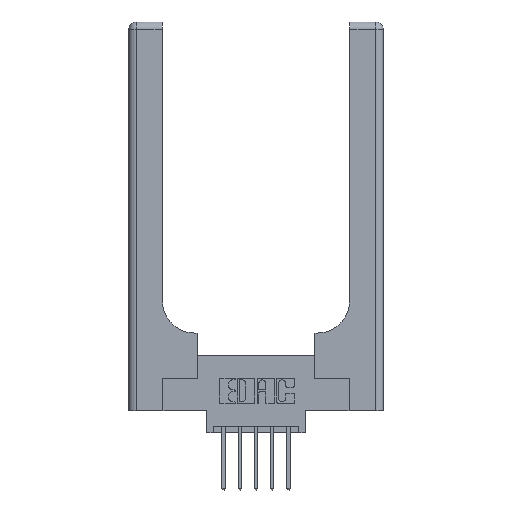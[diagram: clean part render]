
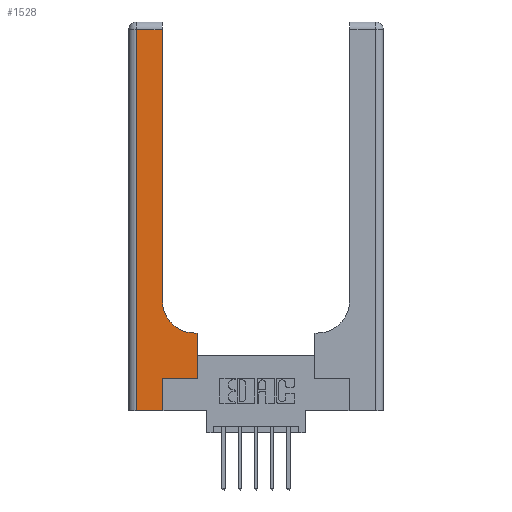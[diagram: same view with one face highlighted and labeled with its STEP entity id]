
A CAD part, top view. The second image highlights one B-rep face of the part: STEP entity #1528.
In plain terms, the highlighted planar face has unit normal (0, 0, 1).
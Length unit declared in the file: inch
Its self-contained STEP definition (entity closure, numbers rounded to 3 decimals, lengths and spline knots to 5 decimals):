
#241 = VERTEX_POINT ( 'NONE', #13091 ) ;
#368 = CARTESIAN_POINT ( 'NONE',  ( 0.26, 0.6, 0.37 ) ) ;
#558 = AXIS2_PLACEMENT_3D ( 'NONE', #2887, #4079, #7356 ) ;
#729 = EDGE_CURVE ( 'NONE', #6492, #241, #1515, .T. ) ;
#746 = EDGE_CURVE ( 'NONE', #5342, #8816, #9026, .T. ) ;
#931 = VECTOR ( 'NONE', #11128, 39.37008 ) ;
#939 = VERTEX_POINT ( 'NONE', #9441 ) ;
#1125 = CARTESIAN_POINT ( 'NONE',  ( 0., 2.94, 0.37 ) ) ;
#1515 = LINE ( 'NONE', #6970, #931 ) ;
#1528 = ADVANCED_FACE ( 'NONE', ( #13864 ), #2510, .F. ) ;
#1964 = LINE ( 'NONE', #7212, #5113 ) ;
#2036 = DIRECTION ( 'NONE',  ( 0., 0., -1. ) ) ;
#2058 = CARTESIAN_POINT ( 'NONE',  ( 0.06, 3., 0.37 ) ) ;
#2380 = CARTESIAN_POINT ( 'NONE',  ( 0.26, 3., 0.37 ) ) ;
#2453 = EDGE_CURVE ( 'NONE', #11182, #13626, #10834, .T. ) ;
#2510 = PLANE ( 'NONE',  #11345 ) ;
#2789 = EDGE_LOOP ( 'NONE', ( #8010, #5596, #9227, #6378, #9759, #4719, #12224, #5224, #10819 ) ) ;
#2887 = CARTESIAN_POINT ( 'NONE',  ( 0.51, 0.85, 0.37 ) ) ;
#4079 = DIRECTION ( 'NONE',  ( 0., 0., -1. ) ) ;
#4421 = EDGE_CURVE ( 'NONE', #13109, #10190, #1964, .T. ) ;
#4426 = CARTESIAN_POINT ( 'NONE',  ( 0.265, 0., 0.37 ) ) ;
#4457 = CARTESIAN_POINT ( 'NONE',  ( 0.51, 0.6, 0.37 ) ) ;
#4687 = EDGE_CURVE ( 'NONE', #939, #11182, #5651, .T. ) ;
#4712 = DIRECTION ( 'NONE',  ( 0., 1., 0. ) ) ;
#4719 = ORIENTED_EDGE ( 'NONE', *, *, #729, .T. ) ;
#4799 = VECTOR ( 'NONE', #5470, 39.37008 ) ;
#5113 = VECTOR ( 'NONE', #13652, 39.37008 ) ;
#5189 = CARTESIAN_POINT ( 'NONE',  ( 0.06, 0., 0.37 ) ) ;
#5224 = ORIENTED_EDGE ( 'NONE', *, *, #746, .T. ) ;
#5342 = VERTEX_POINT ( 'NONE', #6274 ) ;
#5470 = DIRECTION ( 'NONE',  ( 0., -1., 0. ) ) ;
#5596 = ORIENTED_EDGE ( 'NONE', *, *, #2453, .T. ) ;
#5651 = LINE ( 'NONE', #2380, #13481 ) ;
#5826 = DIRECTION ( 'NONE',  ( -1., 0., 0. ) ) ;
#6274 = CARTESIAN_POINT ( 'NONE',  ( 0.528, 0.6, 0.37 ) ) ;
#6378 = ORIENTED_EDGE ( 'NONE', *, *, #4421, .T. ) ;
#6492 = VERTEX_POINT ( 'NONE', #9311 ) ;
#6605 = LINE ( 'NONE', #12118, #6764 ) ;
#6692 = CIRCLE ( 'NONE', #558, 0.25 ) ;
#6764 = VECTOR ( 'NONE', #10903, 39.37008 ) ;
#6970 = CARTESIAN_POINT ( 'NONE',  ( 0.265, 0.25, 0.37 ) ) ;
#7134 = EDGE_CURVE ( 'NONE', #10190, #6492, #11827, .T. ) ;
#7212 = CARTESIAN_POINT ( 'NONE',  ( 0., 0., 0.37 ) ) ;
#7356 = DIRECTION ( 'NONE',  ( 1., 0., 0. ) ) ;
#7457 = CARTESIAN_POINT ( 'NONE',  ( 0.265, 0., 0.37 ) ) ;
#7591 = LINE ( 'NONE', #2058, #4799 ) ;
#7633 = CARTESIAN_POINT ( 'NONE',  ( 0.06, 2.94, 0.37 ) ) ;
#8010 = ORIENTED_EDGE ( 'NONE', *, *, #4687, .T. ) ;
#8470 = EDGE_CURVE ( 'NONE', #241, #5342, #6605, .T. ) ;
#8695 = CARTESIAN_POINT ( 'NONE',  ( 0., 3., 0.37 ) ) ;
#8816 = VERTEX_POINT ( 'NONE', #4457 ) ;
#9026 = LINE ( 'NONE', #368, #11570 ) ;
#9227 = ORIENTED_EDGE ( 'NONE', *, *, #12174, .T. ) ;
#9229 = DIRECTION ( 'NONE',  ( -1., 0., 0. ) ) ;
#9311 = CARTESIAN_POINT ( 'NONE',  ( 0.265, 0.25, 0.37 ) ) ;
#9441 = CARTESIAN_POINT ( 'NONE',  ( 0.26, 0.85, 0.37 ) ) ;
#9759 = ORIENTED_EDGE ( 'NONE', *, *, #7134, .T. ) ;
#10190 = VERTEX_POINT ( 'NONE', #4426 ) ;
#10464 = VECTOR ( 'NONE', #5826, 39.37008 ) ;
#10819 = ORIENTED_EDGE ( 'NONE', *, *, #11226, .T. ) ;
#10834 = LINE ( 'NONE', #1125, #10464 ) ;
#10903 = DIRECTION ( 'NONE',  ( 0., 1., 0. ) ) ;
#11128 = DIRECTION ( 'NONE',  ( 1., 0., 0. ) ) ;
#11182 = VERTEX_POINT ( 'NONE', #13581 ) ;
#11226 = EDGE_CURVE ( 'NONE', #8816, #939, #6692, .T. ) ;
#11345 = AXIS2_PLACEMENT_3D ( 'NONE', #8695, #2036, #11742 ) ;
#11570 = VECTOR ( 'NONE', #9229, 39.37008 ) ;
#11742 = DIRECTION ( 'NONE',  ( -1., 0., 0. ) ) ;
#11827 = LINE ( 'NONE', #7457, #13675 ) ;
#12118 = CARTESIAN_POINT ( 'NONE',  ( 0.528, 0.25, 0.37 ) ) ;
#12174 = EDGE_CURVE ( 'NONE', #13626, #13109, #7591, .T. ) ;
#12224 = ORIENTED_EDGE ( 'NONE', *, *, #8470, .T. ) ;
#12832 = DIRECTION ( 'NONE',  ( 0., 1., 0. ) ) ;
#13091 = CARTESIAN_POINT ( 'NONE',  ( 0.528, 0.25, 0.37 ) ) ;
#13109 = VERTEX_POINT ( 'NONE', #5189 ) ;
#13481 = VECTOR ( 'NONE', #4712, 39.37008 ) ;
#13581 = CARTESIAN_POINT ( 'NONE',  ( 0.26, 2.94, 0.37 ) ) ;
#13626 = VERTEX_POINT ( 'NONE', #7633 ) ;
#13652 = DIRECTION ( 'NONE',  ( 1., 0., 0. ) ) ;
#13675 = VECTOR ( 'NONE', #12832, 39.37008 ) ;
#13864 = FACE_OUTER_BOUND ( 'NONE', #2789, .T. ) ;
